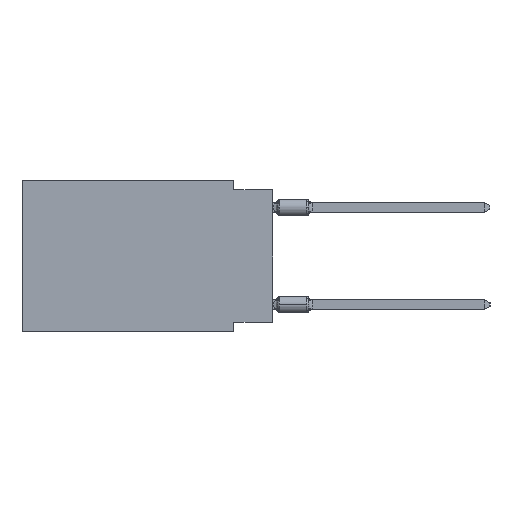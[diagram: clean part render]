
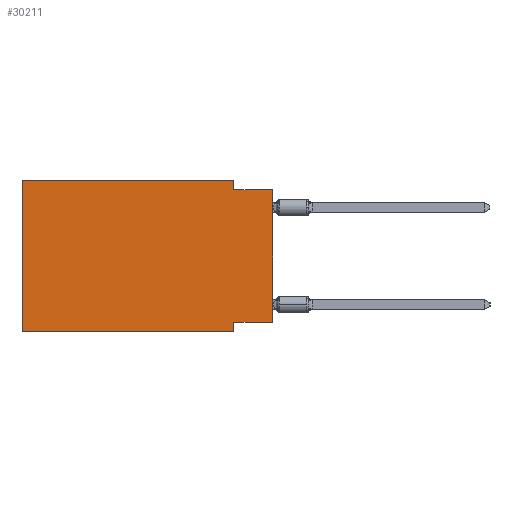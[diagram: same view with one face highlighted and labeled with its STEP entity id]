
A CAD part, left-side view. The second image highlights one B-rep face of the part: STEP entity #30211.
In plain terms, the highlighted planar face has unit normal (-1, 0, 0).
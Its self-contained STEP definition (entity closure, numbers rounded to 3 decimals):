
#661 = VERTEX_POINT ( 'NONE', #51563 ) ;
#1132 = LINE ( 'NONE', #38552, #52889 ) ;
#2272 = LINE ( 'NONE', #15266, #4502 ) ;
#3055 = VECTOR ( 'NONE', #18905, 1000. ) ;
#3094 = VECTOR ( 'NONE', #5469, 1000. ) ;
#4108 = LINE ( 'NONE', #17341, #15672 ) ;
#4502 = VECTOR ( 'NONE', #31805, 1000. ) ;
#5469 = DIRECTION ( 'NONE',  ( 0., 0., 1. ) ) ;
#7063 = EDGE_CURVE ( 'NONE', #48879, #49181, #17833, .T. ) ;
#7559 = EDGE_CURVE ( 'NONE', #9731, #51240, #2272, .T. ) ;
#7997 = LINE ( 'NONE', #50757, #3094 ) ;
#9578 = CARTESIAN_POINT ( 'NONE',  ( 0., 0., -0.635 ) ) ;
#9725 = CARTESIAN_POINT ( 'NONE',  ( 0., 16.383, 0. ) ) ;
#9731 = VERTEX_POINT ( 'NONE', #36080 ) ;
#11368 = EDGE_CURVE ( 'NONE', #24013, #51862, #38471, .T. ) ;
#11475 = EDGE_CURVE ( 'NONE', #24013, #51240, #49039, .T. ) ;
#11949 = ORIENTED_EDGE ( 'NONE', *, *, #25665, .F. ) ;
#11991 = EDGE_CURVE ( 'NONE', #661, #49181, #7997, .T. ) ;
#12012 = ORIENTED_EDGE ( 'NONE', *, *, #11475, .T. ) ;
#12758 = DIRECTION ( 'NONE',  ( 0., 1., 0. ) ) ;
#13016 = LINE ( 'NONE', #28760, #28936 ) ;
#15266 = CARTESIAN_POINT ( 'NONE',  ( 0., 2.54, -9.906 ) ) ;
#15672 = VECTOR ( 'NONE', #20893, 1000. ) ;
#15745 = CARTESIAN_POINT ( 'NONE',  ( 0., 16.383, -9.906 ) ) ;
#16229 = EDGE_LOOP ( 'NONE', ( #24098, #23097, #11949, #43809, #46326, #12012, #48029, #17835 ) ) ;
#16872 = VECTOR ( 'NONE', #50947, 1000. ) ;
#17341 = CARTESIAN_POINT ( 'NONE',  ( 0., 2.54, 0. ) ) ;
#17687 = CARTESIAN_POINT ( 'NONE',  ( 0., 16.383, 0. ) ) ;
#17833 = LINE ( 'NONE', #46072, #47775 ) ;
#17835 = ORIENTED_EDGE ( 'NONE', *, *, #47035, .F. ) ;
#17948 = DIRECTION ( 'NONE',  ( 0., 0., -1. ) ) ;
#18905 = DIRECTION ( 'NONE',  ( 0., -1., 0. ) ) ;
#20893 = DIRECTION ( 'NONE',  ( 0., 0., -1. ) ) ;
#23097 = ORIENTED_EDGE ( 'NONE', *, *, #7063, .F. ) ;
#23757 = EDGE_CURVE ( 'NONE', #51862, #26737, #1132, .T. ) ;
#23976 = CARTESIAN_POINT ( 'NONE',  ( 0., 2.54, 0. ) ) ;
#24013 = VERTEX_POINT ( 'NONE', #15745 ) ;
#24098 = ORIENTED_EDGE ( 'NONE', *, *, #11991, .T. ) ;
#25665 = EDGE_CURVE ( 'NONE', #26737, #48879, #4108, .T. ) ;
#26737 = VERTEX_POINT ( 'NONE', #23976 ) ;
#28398 = CARTESIAN_POINT ( 'NONE',  ( 0., 16.383, -9.906 ) ) ;
#28445 = AXIS2_PLACEMENT_3D ( 'NONE', #17687, #34789, #17948 ) ;
#28760 = CARTESIAN_POINT ( 'NONE',  ( 0., 0., -9.271 ) ) ;
#28936 = VECTOR ( 'NONE', #12758, 1000. ) ;
#30211 = ADVANCED_FACE ( 'NONE', ( #43192 ), #38587, .F. ) ;
#31805 = DIRECTION ( 'NONE',  ( 0., 0., -1. ) ) ;
#33773 = CARTESIAN_POINT ( 'NONE',  ( 0., 2.54, -0.635 ) ) ;
#34789 = DIRECTION ( 'NONE',  ( 1., 0., 0. ) ) ;
#36080 = CARTESIAN_POINT ( 'NONE',  ( 0., 2.54, -9.271 ) ) ;
#36882 = CARTESIAN_POINT ( 'NONE',  ( 0., 2.54, -9.906 ) ) ;
#37916 = DIRECTION ( 'NONE',  ( 0., -1., 0. ) ) ;
#38471 = LINE ( 'NONE', #9725, #16872 ) ;
#38552 = CARTESIAN_POINT ( 'NONE',  ( 0., 16.383, 0. ) ) ;
#38587 = PLANE ( 'NONE',  #28445 ) ;
#43192 = FACE_OUTER_BOUND ( 'NONE', #16229, .T. ) ;
#43809 = ORIENTED_EDGE ( 'NONE', *, *, #23757, .F. ) ;
#46072 = CARTESIAN_POINT ( 'NONE',  ( 0., 0., -0.635 ) ) ;
#46326 = ORIENTED_EDGE ( 'NONE', *, *, #11368, .F. ) ;
#46685 = DIRECTION ( 'NONE',  ( 0., -1., 0. ) ) ;
#47035 = EDGE_CURVE ( 'NONE', #661, #9731, #13016, .T. ) ;
#47361 = CARTESIAN_POINT ( 'NONE',  ( 0., 16.383, 0. ) ) ;
#47775 = VECTOR ( 'NONE', #37916, 1000. ) ;
#48029 = ORIENTED_EDGE ( 'NONE', *, *, #7559, .F. ) ;
#48879 = VERTEX_POINT ( 'NONE', #33773 ) ;
#49039 = LINE ( 'NONE', #28398, #3055 ) ;
#49181 = VERTEX_POINT ( 'NONE', #9578 ) ;
#50757 = CARTESIAN_POINT ( 'NONE',  ( 0., 0., 0. ) ) ;
#50947 = DIRECTION ( 'NONE',  ( 0., 0., 1. ) ) ;
#51240 = VERTEX_POINT ( 'NONE', #36882 ) ;
#51563 = CARTESIAN_POINT ( 'NONE',  ( 0., 0., -9.271 ) ) ;
#51862 = VERTEX_POINT ( 'NONE', #47361 ) ;
#52889 = VECTOR ( 'NONE', #46685, 1000. ) ;
